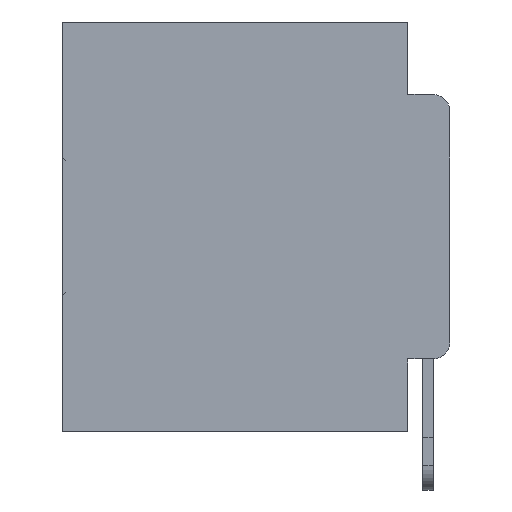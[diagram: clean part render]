
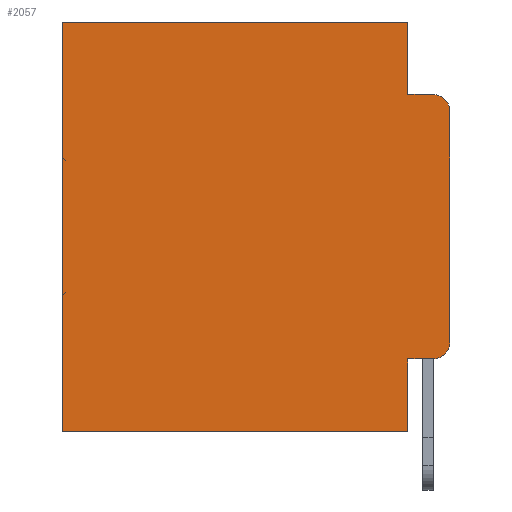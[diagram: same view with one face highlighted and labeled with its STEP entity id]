
A CAD part, left-side view. The second image highlights one B-rep face of the part: STEP entity #2057.
In plain terms, the highlighted planar face has unit normal (-1, 0, 0).
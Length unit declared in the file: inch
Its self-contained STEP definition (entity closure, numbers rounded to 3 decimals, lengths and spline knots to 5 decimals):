
#101 = LINE ( 'NONE', #27109, #25865 ) ;
#272 = CARTESIAN_POINT ( 'NONE',  ( 0.298, 0., -0.3915 ) ) ;
#504 = CARTESIAN_POINT ( 'NONE',  ( 0.298, 0.473, 0. ) ) ;
#572 = DIRECTION ( 'NONE',  ( 0., 0., -1. ) ) ;
#582 = ORIENTED_EDGE ( 'NONE', *, *, #24386, .T. ) ;
#1700 = CARTESIAN_POINT ( 'NONE',  ( 0.298, 0., 0. ) ) ;
#2057 = ADVANCED_FACE ( 'NONE', ( #6805 ), #30327, .F. ) ;
#2957 = CARTESIAN_POINT ( 'NONE',  ( 0.298, 0., -0.1085 ) ) ;
#3082 = DIRECTION ( 'NONE',  ( 1., 0., 0. ) ) ;
#3193 = CARTESIAN_POINT ( 'NONE',  ( 0.298, 0.051, 0. ) ) ;
#3549 = AXIS2_PLACEMENT_3D ( 'NONE', #13693, #30762, #16194 ) ;
#3885 = DIRECTION ( 'NONE',  ( 0., -1., 0. ) ) ;
#4020 = VERTEX_POINT ( 'NONE', #14387 ) ;
#5112 = VERTEX_POINT ( 'NONE', #8407 ) ;
#5494 = EDGE_CURVE ( 'NONE', #5112, #14467, #101, .T. ) ;
#5678 = CARTESIAN_POINT ( 'NONE',  ( 0.298, 0.02, -0.4115 ) ) ;
#6404 = CARTESIAN_POINT ( 'NONE',  ( 0.298, 0.02, -0.1085 ) ) ;
#6430 = LINE ( 'NONE', #16411, #25395 ) ;
#6734 = AXIS2_PLACEMENT_3D ( 'NONE', #6404, #23735, #8958 ) ;
#6805 = FACE_OUTER_BOUND ( 'NONE', #20281, .T. ) ;
#8010 = EDGE_CURVE ( 'NONE', #19548, #27517, #17931, .T. ) ;
#8407 = CARTESIAN_POINT ( 'NONE',  ( 0.298, 0.051, -0.4115 ) ) ;
#8892 = EDGE_CURVE ( 'NONE', #14467, #17502, #14019, .T. ) ;
#8958 = DIRECTION ( 'NONE',  ( 0., 0., -1. ) ) ;
#10400 = DIRECTION ( 'NONE',  ( 0., 0., -1. ) ) ;
#10797 = EDGE_CURVE ( 'NONE', #28328, #27517, #6430, .T. ) ;
#10945 = DIRECTION ( 'NONE',  ( 0., 1., 0. ) ) ;
#11229 = EDGE_CURVE ( 'NONE', #4020, #28328, #26875, .T. ) ;
#11758 = ORIENTED_EDGE ( 'NONE', *, *, #8010, .T. ) ;
#13621 = EDGE_CURVE ( 'NONE', #19548, #17502, #30641, .T. ) ;
#13693 = CARTESIAN_POINT ( 'NONE',  ( 0.298, 0.02, -0.3915 ) ) ;
#14019 = CIRCLE ( 'NONE', #3549, 0.02 ) ;
#14387 = CARTESIAN_POINT ( 'NONE',  ( 0.298, 0.051, 0. ) ) ;
#14467 = VERTEX_POINT ( 'NONE', #5678 ) ;
#14806 = VERTEX_POINT ( 'NONE', #19699 ) ;
#15079 = VECTOR ( 'NONE', #15587, 39.37008 ) ;
#15587 = DIRECTION ( 'NONE',  ( 0., 1., 0. ) ) ;
#16194 = DIRECTION ( 'NONE',  ( 0., 0., -1. ) ) ;
#16411 = CARTESIAN_POINT ( 'NONE',  ( 0.298, 0.051, -0.0885 ) ) ;
#16700 = DIRECTION ( 'NONE',  ( 0., 0., -1. ) ) ;
#17502 = VERTEX_POINT ( 'NONE', #272 ) ;
#17719 = VECTOR ( 'NONE', #26689, 39.37008 ) ;
#17931 = CIRCLE ( 'NONE', #6734, 0.02 ) ;
#19548 = VERTEX_POINT ( 'NONE', #2957 ) ;
#19699 = CARTESIAN_POINT ( 'NONE',  ( 0.298, 0.051, -0.5 ) ) ;
#19834 = ORIENTED_EDGE ( 'NONE', *, *, #11229, .F. ) ;
#20177 = CARTESIAN_POINT ( 'NONE',  ( 0.298, 0.473, 0. ) ) ;
#20281 = EDGE_LOOP ( 'NONE', ( #23266, #11758, #31235, #19834, #26340, #582, #27077, #21360, #29349, #23677 ) ) ;
#21360 = ORIENTED_EDGE ( 'NONE', *, *, #27624, .F. ) ;
#21578 = LINE ( 'NONE', #25288, #15079 ) ;
#22145 = EDGE_CURVE ( 'NONE', #14806, #29955, #21578, .T. ) ;
#22180 = VERTEX_POINT ( 'NONE', #504 ) ;
#22226 = DIRECTION ( 'NONE',  ( 0., -1., 0. ) ) ;
#23266 = ORIENTED_EDGE ( 'NONE', *, *, #13621, .F. ) ;
#23379 = VECTOR ( 'NONE', #10945, 39.37008 ) ;
#23525 = CARTESIAN_POINT ( 'NONE',  ( 0.298, 0.02, -0.0885 ) ) ;
#23677 = ORIENTED_EDGE ( 'NONE', *, *, #8892, .T. ) ;
#23735 = DIRECTION ( 'NONE',  ( -1., 0., 0. ) ) ;
#24262 = VECTOR ( 'NONE', #10400, 39.37008 ) ;
#24386 = EDGE_CURVE ( 'NONE', #22180, #29955, #30677, .T. ) ;
#24961 = LINE ( 'NONE', #31242, #25702 ) ;
#25288 = CARTESIAN_POINT ( 'NONE',  ( 0.298, 0., -0.5 ) ) ;
#25395 = VECTOR ( 'NONE', #3885, 39.37008 ) ;
#25449 = AXIS2_PLACEMENT_3D ( 'NONE', #27882, #3082, #572 ) ;
#25568 = DIRECTION ( 'NONE',  ( 0., 0., -1. ) ) ;
#25702 = VECTOR ( 'NONE', #16700, 39.37008 ) ;
#25865 = VECTOR ( 'NONE', #22226, 39.37008 ) ;
#26126 = VECTOR ( 'NONE', #25568, 39.37008 ) ;
#26340 = ORIENTED_EDGE ( 'NONE', *, *, #28080, .T. ) ;
#26567 = CARTESIAN_POINT ( 'NONE',  ( 0.298, 0.051, -0.0885 ) ) ;
#26689 = DIRECTION ( 'NONE',  ( 0., 0., -1. ) ) ;
#26875 = LINE ( 'NONE', #3193, #26126 ) ;
#27077 = ORIENTED_EDGE ( 'NONE', *, *, #22145, .F. ) ;
#27109 = CARTESIAN_POINT ( 'NONE',  ( 0.298, 0.051, -0.4115 ) ) ;
#27517 = VERTEX_POINT ( 'NONE', #23525 ) ;
#27624 = EDGE_CURVE ( 'NONE', #5112, #14806, #24961, .T. ) ;
#27882 = CARTESIAN_POINT ( 'NONE',  ( 0.298, 0., 0. ) ) ;
#27941 = CARTESIAN_POINT ( 'NONE',  ( 0.298, 0., 0. ) ) ;
#28080 = EDGE_CURVE ( 'NONE', #4020, #22180, #30584, .T. ) ;
#28328 = VERTEX_POINT ( 'NONE', #26567 ) ;
#29133 = CARTESIAN_POINT ( 'NONE',  ( 0.298, 0.473, -0.5 ) ) ;
#29349 = ORIENTED_EDGE ( 'NONE', *, *, #5494, .T. ) ;
#29955 = VERTEX_POINT ( 'NONE', #29133 ) ;
#30327 = PLANE ( 'NONE',  #25449 ) ;
#30584 = LINE ( 'NONE', #27941, #23379 ) ;
#30641 = LINE ( 'NONE', #1700, #17719 ) ;
#30677 = LINE ( 'NONE', #20177, #24262 ) ;
#30762 = DIRECTION ( 'NONE',  ( -1., 0., 0. ) ) ;
#31235 = ORIENTED_EDGE ( 'NONE', *, *, #10797, .F. ) ;
#31242 = CARTESIAN_POINT ( 'NONE',  ( 0.298, 0.051, 0. ) ) ;
